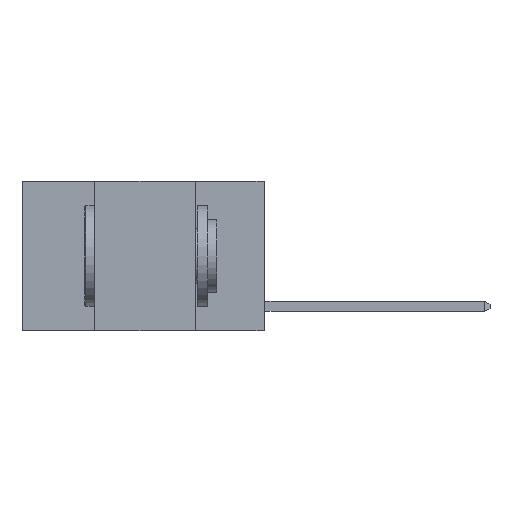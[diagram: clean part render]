
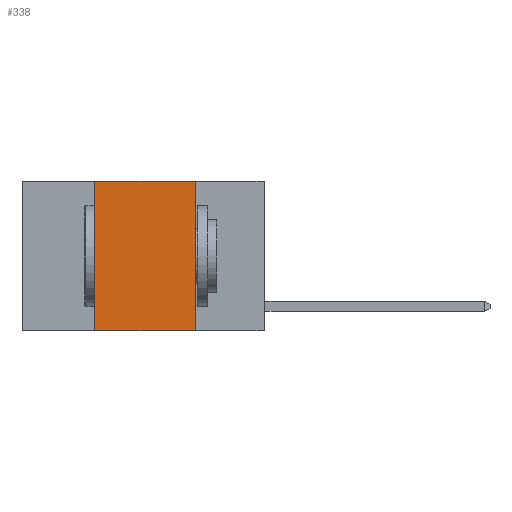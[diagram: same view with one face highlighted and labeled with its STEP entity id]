
A CAD part, left-side view. The second image highlights one B-rep face of the part: STEP entity #338.
In plain terms, the highlighted planar face has unit normal (-1, 0, 0).
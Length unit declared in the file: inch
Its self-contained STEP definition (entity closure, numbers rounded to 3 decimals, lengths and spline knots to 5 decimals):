
#338 = ADVANCED_FACE ( 'NONE', ( #711 ), #2120, .F. ) ;
#479 = CARTESIAN_POINT ( 'NONE',  ( 0., 0.6, -0.37 ) ) ;
#667 = ORIENTED_EDGE ( 'NONE', *, *, #1804, .F. ) ;
#711 = FACE_OUTER_BOUND ( 'NONE', #1970, .T. ) ;
#818 = LINE ( 'NONE', #5120, #7969 ) ;
#888 = ORIENTED_EDGE ( 'NONE', *, *, #3717, .T. ) ;
#1050 = VERTEX_POINT ( 'NONE', #1835 ) ;
#1289 = CARTESIAN_POINT ( 'NONE',  ( 0., 0.17, -0.37 ) ) ;
#1403 = VERTEX_POINT ( 'NONE', #1289 ) ;
#1804 = EDGE_CURVE ( 'NONE', #2454, #3798, #818, .T. ) ;
#1835 = CARTESIAN_POINT ( 'NONE',  ( 0., 0.17, 0. ) ) ;
#1950 = DIRECTION ( 'NONE',  ( 0., -1., 0. ) ) ;
#1970 = EDGE_LOOP ( 'NONE', ( #3098, #3606, #667, #888 ) ) ;
#2119 = VECTOR ( 'NONE', #1950, 39.37008 ) ;
#2120 = PLANE ( 'NONE',  #3928 ) ;
#2454 = VERTEX_POINT ( 'NONE', #5683 ) ;
#2685 = DIRECTION ( 'NONE',  ( 0., 0., -1. ) ) ;
#3084 = LINE ( 'NONE', #5865, #5146 ) ;
#3098 = ORIENTED_EDGE ( 'NONE', *, *, #4362, .F. ) ;
#3194 = LINE ( 'NONE', #6796, #4588 ) ;
#3606 = ORIENTED_EDGE ( 'NONE', *, *, #4073, .F. ) ;
#3717 = EDGE_CURVE ( 'NONE', #2454, #1403, #4049, .T. ) ;
#3798 = VERTEX_POINT ( 'NONE', #5570 ) ;
#3928 = AXIS2_PLACEMENT_3D ( 'NONE', #7731, #5814, #7211 ) ;
#4049 = LINE ( 'NONE', #479, #2119 ) ;
#4073 = EDGE_CURVE ( 'NONE', #3798, #1050, #3084, .T. ) ;
#4362 = EDGE_CURVE ( 'NONE', #1050, #1403, #3194, .T. ) ;
#4588 = VECTOR ( 'NONE', #2685, 39.37008 ) ;
#4923 = DIRECTION ( 'NONE',  ( 0., 0., 1. ) ) ;
#5120 = CARTESIAN_POINT ( 'NONE',  ( 0., 0.42, 0. ) ) ;
#5146 = VECTOR ( 'NONE', #7832, 39.37008 ) ;
#5570 = CARTESIAN_POINT ( 'NONE',  ( 0., 0.42, 0. ) ) ;
#5683 = CARTESIAN_POINT ( 'NONE',  ( 0., 0.42, -0.37 ) ) ;
#5814 = DIRECTION ( 'NONE',  ( 1., 0., 0. ) ) ;
#5865 = CARTESIAN_POINT ( 'NONE',  ( 0., 0.6, 0. ) ) ;
#6796 = CARTESIAN_POINT ( 'NONE',  ( 0., 0.17, 0. ) ) ;
#7211 = DIRECTION ( 'NONE',  ( 0., 0., -1. ) ) ;
#7731 = CARTESIAN_POINT ( 'NONE',  ( 0., 0.6, 0. ) ) ;
#7832 = DIRECTION ( 'NONE',  ( 0., -1., 0. ) ) ;
#7969 = VECTOR ( 'NONE', #4923, 39.37008 ) ;
